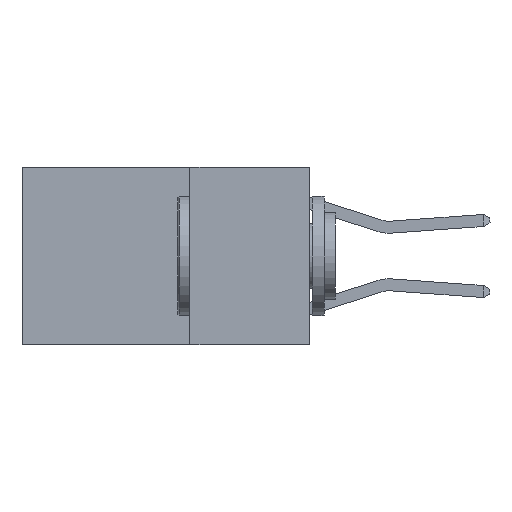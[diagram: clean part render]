
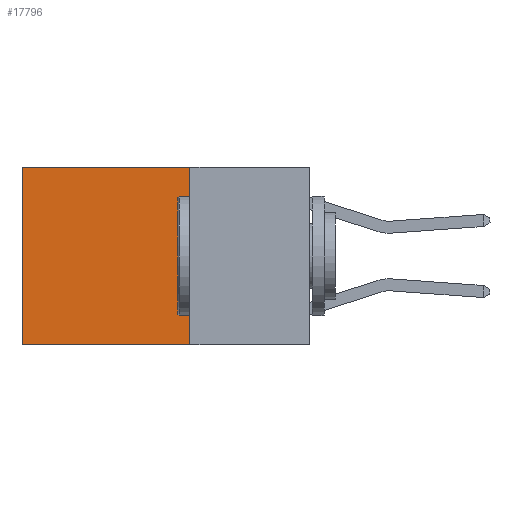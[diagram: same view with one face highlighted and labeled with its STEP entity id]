
A CAD part, left-side view. The second image highlights one B-rep face of the part: STEP entity #17796.
In plain terms, the highlighted planar face has unit normal (-1, 0, 0).
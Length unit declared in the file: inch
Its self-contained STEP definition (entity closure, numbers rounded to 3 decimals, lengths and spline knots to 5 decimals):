
#1031 = EDGE_CURVE ( 'NONE', #6861, #19983, #16758, .T. ) ;
#1403 = CARTESIAN_POINT ( 'NONE',  ( 0.2625, 0.25, 0. ) ) ;
#1757 = CARTESIAN_POINT ( 'NONE',  ( 0.2625, 0.6, -0.37 ) ) ;
#2792 = DIRECTION ( 'NONE',  ( 1., 0., 0. ) ) ;
#3445 = CARTESIAN_POINT ( 'NONE',  ( 0.2625, 0.25, -0.37 ) ) ;
#4335 = VERTEX_POINT ( 'NONE', #1757 ) ;
#4725 = ORIENTED_EDGE ( 'NONE', *, *, #1031, .F. ) ;
#4776 = CARTESIAN_POINT ( 'NONE',  ( 0.2625, 0.25, 0. ) ) ;
#4828 = EDGE_LOOP ( 'NONE', ( #7649, #7445, #4725, #18799 ) ) ;
#5484 = VERTEX_POINT ( 'NONE', #6744 ) ;
#6744 = CARTESIAN_POINT ( 'NONE',  ( 0.2625, 0.6, 0. ) ) ;
#6861 = VERTEX_POINT ( 'NONE', #1403 ) ;
#7088 = FACE_OUTER_BOUND ( 'NONE', #4828, .T. ) ;
#7445 = ORIENTED_EDGE ( 'NONE', *, *, #14412, .F. ) ;
#7649 = ORIENTED_EDGE ( 'NONE', *, *, #17041, .T. ) ;
#10227 = PLANE ( 'NONE',  #21811 ) ;
#11325 = LINE ( 'NONE', #16004, #20583 ) ;
#11865 = VECTOR ( 'NONE', #16952, 39.37008 ) ;
#14057 = LINE ( 'NONE', #17760, #23855 ) ;
#14412 = EDGE_CURVE ( 'NONE', #19983, #4335, #11325, .T. ) ;
#14707 = LINE ( 'NONE', #4776, #18478 ) ;
#15653 = EDGE_CURVE ( 'NONE', #6861, #5484, #14707, .T. ) ;
#15787 = DIRECTION ( 'NONE',  ( 0., 0., -1. ) ) ;
#16004 = CARTESIAN_POINT ( 'NONE',  ( 0.2625, 0.25, -0.37 ) ) ;
#16758 = LINE ( 'NONE', #17481, #11865 ) ;
#16952 = DIRECTION ( 'NONE',  ( 0., 0., -1. ) ) ;
#17041 = EDGE_CURVE ( 'NONE', #5484, #4335, #14057, .T. ) ;
#17481 = CARTESIAN_POINT ( 'NONE',  ( 0.2625, 0.25, 0. ) ) ;
#17760 = CARTESIAN_POINT ( 'NONE',  ( 0.2625, 0.6, 0. ) ) ;
#17796 = ADVANCED_FACE ( 'NONE', ( #7088 ), #10227, .F. ) ;
#17865 = DIRECTION ( 'NONE',  ( 0., 1., 0. ) ) ;
#18478 = VECTOR ( 'NONE', #21462, 39.37008 ) ;
#18799 = ORIENTED_EDGE ( 'NONE', *, *, #15653, .T. ) ;
#19440 = CARTESIAN_POINT ( 'NONE',  ( 0.2625, 0.25, 0. ) ) ;
#19628 = DIRECTION ( 'NONE',  ( 0., 0., -1. ) ) ;
#19983 = VERTEX_POINT ( 'NONE', #3445 ) ;
#20583 = VECTOR ( 'NONE', #17865, 39.37008 ) ;
#21462 = DIRECTION ( 'NONE',  ( 0., 1., 0. ) ) ;
#21811 = AXIS2_PLACEMENT_3D ( 'NONE', #19440, #2792, #15787 ) ;
#23855 = VECTOR ( 'NONE', #19628, 39.37008 ) ;
